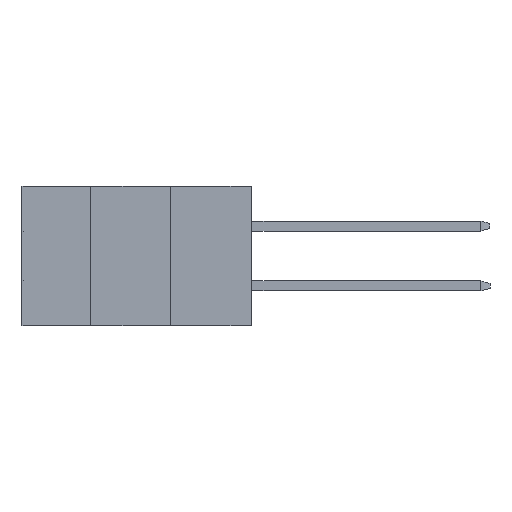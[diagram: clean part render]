
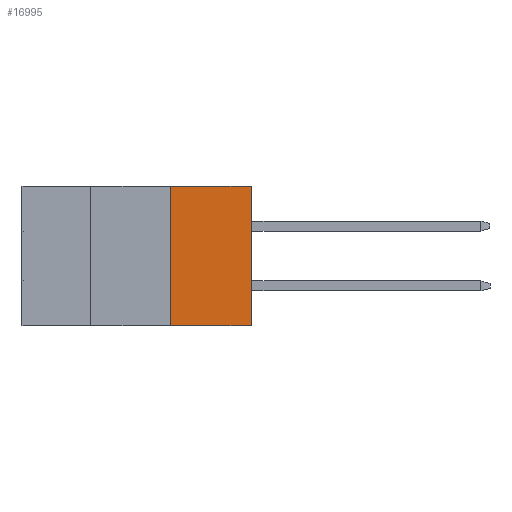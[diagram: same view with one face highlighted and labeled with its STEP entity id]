
A CAD part, left-side view. The second image highlights one B-rep face of the part: STEP entity #16995.
In plain terms, the highlighted planar face has unit normal (-1, 0, 0).
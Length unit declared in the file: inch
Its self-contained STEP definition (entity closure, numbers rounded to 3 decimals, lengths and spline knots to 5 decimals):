
#107 = LINE ( 'NONE', #21213, #19238 ) ;
#134 = EDGE_CURVE ( 'NONE', #13460, #21515, #107, .T. ) ;
#1026 = DIRECTION ( 'NONE',  ( 0., 0., 1. ) ) ;
#1425 = AXIS2_PLACEMENT_3D ( 'NONE', #2729, #21307, #10983 ) ;
#1847 = CARTESIAN_POINT ( 'NONE',  ( 0.4265, 0.254, 0. ) ) ;
#2618 = FACE_OUTER_BOUND ( 'NONE', #4450, .T. ) ;
#2729 = CARTESIAN_POINT ( 'NONE',  ( 0.4265, 0.254, -0.437 ) ) ;
#4450 = EDGE_LOOP ( 'NONE', ( #6241, #15422, #16139, #19119 ) ) ;
#4748 = VECTOR ( 'NONE', #18131, 39.37008 ) ;
#5309 = VERTEX_POINT ( 'NONE', #1847 ) ;
#5878 = DIRECTION ( 'NONE',  ( 0., -1., 0. ) ) ;
#6241 = ORIENTED_EDGE ( 'NONE', *, *, #10980, .T. ) ;
#6488 = CARTESIAN_POINT ( 'NONE',  ( 0.4265, 0.254, 0. ) ) ;
#7358 = VERTEX_POINT ( 'NONE', #12814 ) ;
#7694 = CARTESIAN_POINT ( 'NONE',  ( 0.4265, 0.254, -0.437 ) ) ;
#9773 = CARTESIAN_POINT ( 'NONE',  ( 0.4265, 0., -0.437 ) ) ;
#10287 = LINE ( 'NONE', #14170, #11096 ) ;
#10980 = EDGE_CURVE ( 'NONE', #21515, #7358, #14836, .T. ) ;
#10983 = DIRECTION ( 'NONE',  ( 0., 0., -1. ) ) ;
#11096 = VECTOR ( 'NONE', #22062, 39.37008 ) ;
#11455 = VECTOR ( 'NONE', #1026, 39.37008 ) ;
#12814 = CARTESIAN_POINT ( 'NONE',  ( 0.4265, 0., 0. ) ) ;
#13406 = EDGE_CURVE ( 'NONE', #13460, #5309, #10287, .T. ) ;
#13460 = VERTEX_POINT ( 'NONE', #7694 ) ;
#14170 = CARTESIAN_POINT ( 'NONE',  ( 0.4265, 0.254, -0.437 ) ) ;
#14836 = LINE ( 'NONE', #9773, #11455 ) ;
#15110 = LINE ( 'NONE', #6488, #4748 ) ;
#15358 = EDGE_CURVE ( 'NONE', #5309, #7358, #15110, .T. ) ;
#15422 = ORIENTED_EDGE ( 'NONE', *, *, #15358, .F. ) ;
#16139 = ORIENTED_EDGE ( 'NONE', *, *, #13406, .F. ) ;
#16995 = ADVANCED_FACE ( 'NONE', ( #2618 ), #19284, .F. ) ;
#18131 = DIRECTION ( 'NONE',  ( 0., -1., 0. ) ) ;
#19119 = ORIENTED_EDGE ( 'NONE', *, *, #134, .T. ) ;
#19238 = VECTOR ( 'NONE', #5878, 39.37008 ) ;
#19284 = PLANE ( 'NONE',  #1425 ) ;
#21213 = CARTESIAN_POINT ( 'NONE',  ( 0.4265, 0.254, -0.437 ) ) ;
#21307 = DIRECTION ( 'NONE',  ( 1., 0., 0. ) ) ;
#21515 = VERTEX_POINT ( 'NONE', #21740 ) ;
#21740 = CARTESIAN_POINT ( 'NONE',  ( 0.4265, 0., -0.437 ) ) ;
#22062 = DIRECTION ( 'NONE',  ( 0., 0., 1. ) ) ;
